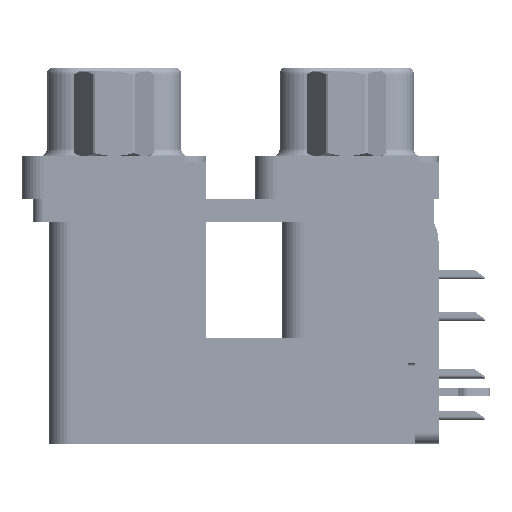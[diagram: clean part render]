
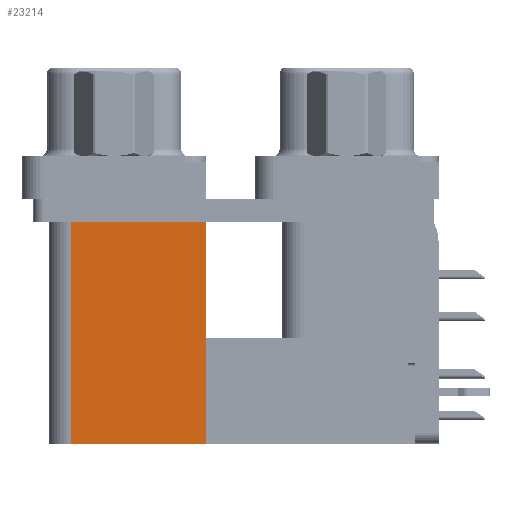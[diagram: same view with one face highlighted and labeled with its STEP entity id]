
A CAD part, left-side view. The second image highlights one B-rep face of the part: STEP entity #23214.
In plain terms, the highlighted planar face has unit normal (-1, 0, 0).
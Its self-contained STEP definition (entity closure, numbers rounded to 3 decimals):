
#157 = CARTESIAN_POINT ( 'NONE',  ( 3.79, 9.6, -2.5 ) ) ;
#805 = CARTESIAN_POINT ( 'NONE',  ( 3.79, 9.6, -19.2 ) ) ;
#1105 = LINE ( 'NONE', #46188, #15998 ) ;
#2672 = LINE ( 'NONE', #38183, #42761 ) ;
#2819 = DIRECTION ( 'NONE',  ( 0., 1., 0. ) ) ;
#5922 = FACE_OUTER_BOUND ( 'NONE', #49273, .T. ) ;
#9079 = CARTESIAN_POINT ( 'NONE',  ( 3.79, 9.6, -2.5 ) ) ;
#11037 = EDGE_CURVE ( 'NONE', #27445, #43216, #2672, .T. ) ;
#11682 = DIRECTION ( 'NONE',  ( 0., 0., 1. ) ) ;
#12123 = LINE ( 'NONE', #29014, #22599 ) ;
#14304 = ORIENTED_EDGE ( 'NONE', *, *, #11037, .T. ) ;
#14662 = CARTESIAN_POINT ( 'NONE',  ( 3.79, 9.6, -19.2 ) ) ;
#15998 = VECTOR ( 'NONE', #18863, 1000. ) ;
#18863 = DIRECTION ( 'NONE',  ( 0., 0., 1. ) ) ;
#22599 = VECTOR ( 'NONE', #2819, 1000. ) ;
#23214 = ADVANCED_FACE ( 'NONE', ( #5922 ), #49592, .F. ) ;
#27445 = VERTEX_POINT ( 'NONE', #805 ) ;
#29014 = CARTESIAN_POINT ( 'NONE',  ( 3.79, 9.6, -19.2 ) ) ;
#34268 = EDGE_CURVE ( 'NONE', #43216, #53819, #34986, .T. ) ;
#34986 = LINE ( 'NONE', #9079, #36768 ) ;
#36585 = ORIENTED_EDGE ( 'NONE', *, *, #53053, .F. ) ;
#36768 = VECTOR ( 'NONE', #57105, 1000. ) ;
#37074 = DIRECTION ( 'NONE',  ( 1., 0., 0. ) ) ;
#37353 = DIRECTION ( 'NONE',  ( 0., 0., -1. ) ) ;
#38183 = CARTESIAN_POINT ( 'NONE',  ( 3.79, 9.6, -19.2 ) ) ;
#42761 = VECTOR ( 'NONE', #11682, 1000. ) ;
#43216 = VERTEX_POINT ( 'NONE', #157 ) ;
#45297 = ORIENTED_EDGE ( 'NONE', *, *, #51443, .F. ) ;
#46188 = CARTESIAN_POINT ( 'NONE',  ( 3.79, 18.8, -19.2 ) ) ;
#47335 = AXIS2_PLACEMENT_3D ( 'NONE', #14662, #37074, #37353 ) ;
#48500 = CARTESIAN_POINT ( 'NONE',  ( 3.79, 18.8, -19.2 ) ) ;
#49273 = EDGE_LOOP ( 'NONE', ( #52657, #45297, #36585, #14304 ) ) ;
#49592 = PLANE ( 'NONE',  #47335 ) ;
#51443 = EDGE_CURVE ( 'NONE', #57079, #53819, #1105, .T. ) ;
#52657 = ORIENTED_EDGE ( 'NONE', *, *, #34268, .T. ) ;
#52785 = CARTESIAN_POINT ( 'NONE',  ( 3.79, 18.8, -2.5 ) ) ;
#53053 = EDGE_CURVE ( 'NONE', #27445, #57079, #12123, .T. ) ;
#53819 = VERTEX_POINT ( 'NONE', #52785 ) ;
#57079 = VERTEX_POINT ( 'NONE', #48500 ) ;
#57105 = DIRECTION ( 'NONE',  ( 0., 1., 0. ) ) ;
